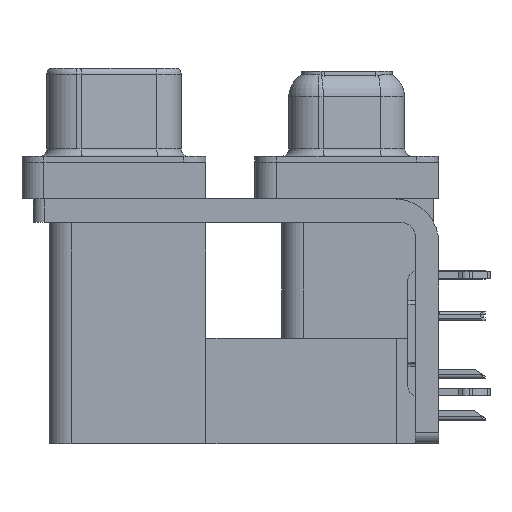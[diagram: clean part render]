
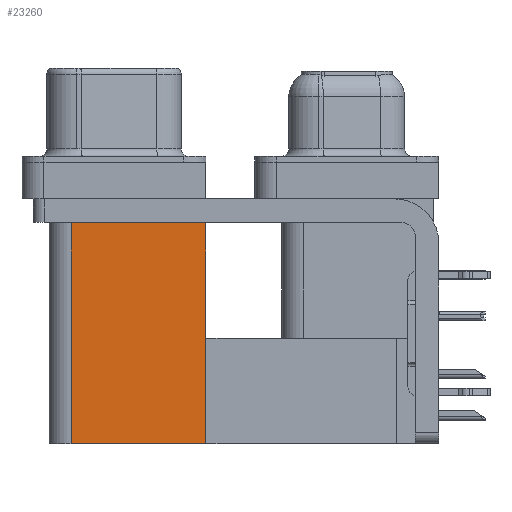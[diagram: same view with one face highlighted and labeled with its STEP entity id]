
A CAD part, left-side view. The second image highlights one B-rep face of the part: STEP entity #23260.
In plain terms, the highlighted planar face has unit normal (-1, 0, 0).
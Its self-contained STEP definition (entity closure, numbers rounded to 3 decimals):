
#594 = ORIENTED_EDGE ( 'NONE', *, *, #656, .F. ) ;
#656 = EDGE_CURVE ( 'NONE', #23495, #26680, #32215, .T. ) ;
#1028 = DIRECTION ( 'NONE',  ( 0., 0., 1. ) ) ;
#1851 = ORIENTED_EDGE ( 'NONE', *, *, #45548, .T. ) ;
#1965 = VECTOR ( 'NONE', #16625, 1000. ) ;
#2603 = VERTEX_POINT ( 'NONE', #45519 ) ;
#3083 = PLANE ( 'NONE',  #28888 ) ;
#4675 = LINE ( 'NONE', #43829, #37224 ) ;
#5213 = EDGE_LOOP ( 'NONE', ( #9157, #594, #19909, #1851 ) ) ;
#5250 = LINE ( 'NONE', #15418, #22627 ) ;
#5788 = LINE ( 'NONE', #40685, #1965 ) ;
#9157 = ORIENTED_EDGE ( 'NONE', *, *, #29238, .T. ) ;
#13712 = FACE_OUTER_BOUND ( 'NONE', #5213, .T. ) ;
#15418 = CARTESIAN_POINT ( 'NONE',  ( 3.765, 9.6, -19.2 ) ) ;
#16625 = DIRECTION ( 'NONE',  ( 0., 1., 0. ) ) ;
#17471 = DIRECTION ( 'NONE',  ( 1., 0., 0. ) ) ;
#18314 = CARTESIAN_POINT ( 'NONE',  ( 3.765, 18.8, -2.5 ) ) ;
#19909 = ORIENTED_EDGE ( 'NONE', *, *, #30520, .F. ) ;
#21931 = CARTESIAN_POINT ( 'NONE',  ( 3.765, 9.6, -19.2 ) ) ;
#22627 = VECTOR ( 'NONE', #1028, 1000. ) ;
#23260 = ADVANCED_FACE ( 'NONE', ( #13712 ), #3083, .F. ) ;
#23495 = VERTEX_POINT ( 'NONE', #27348 ) ;
#24435 = VECTOR ( 'NONE', #25864, 1000. ) ;
#25864 = DIRECTION ( 'NONE',  ( 0., 0., 1. ) ) ;
#26680 = VERTEX_POINT ( 'NONE', #18314 ) ;
#27348 = CARTESIAN_POINT ( 'NONE',  ( 3.765, 18.8, -19.2 ) ) ;
#28888 = AXIS2_PLACEMENT_3D ( 'NONE', #39616, #17471, #32543 ) ;
#29238 = EDGE_CURVE ( 'NONE', #2603, #26680, #4675, .T. ) ;
#29407 = CARTESIAN_POINT ( 'NONE',  ( 3.765, 18.8, -19.2 ) ) ;
#30520 = EDGE_CURVE ( 'NONE', #42057, #23495, #5788, .T. ) ;
#32215 = LINE ( 'NONE', #29407, #24435 ) ;
#32505 = DIRECTION ( 'NONE',  ( 0., 1., 0. ) ) ;
#32543 = DIRECTION ( 'NONE',  ( 0., 0., -1. ) ) ;
#37224 = VECTOR ( 'NONE', #32505, 1000. ) ;
#39616 = CARTESIAN_POINT ( 'NONE',  ( 3.765, 9.6, -19.2 ) ) ;
#40685 = CARTESIAN_POINT ( 'NONE',  ( 3.765, 9.6, -19.2 ) ) ;
#42057 = VERTEX_POINT ( 'NONE', #21931 ) ;
#43829 = CARTESIAN_POINT ( 'NONE',  ( 3.765, 9.6, -2.5 ) ) ;
#45519 = CARTESIAN_POINT ( 'NONE',  ( 3.765, 9.6, -2.5 ) ) ;
#45548 = EDGE_CURVE ( 'NONE', #42057, #2603, #5250, .T. ) ;
